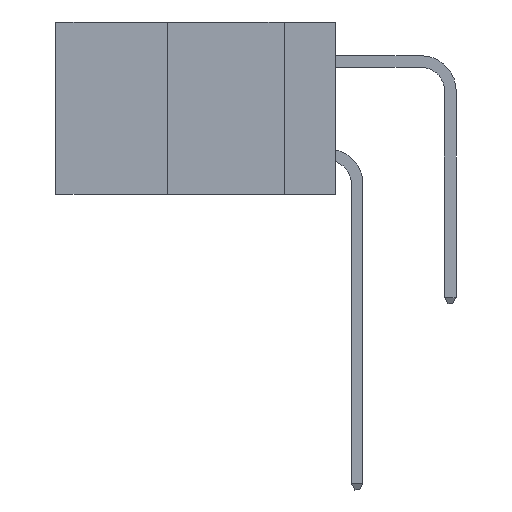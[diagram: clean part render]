
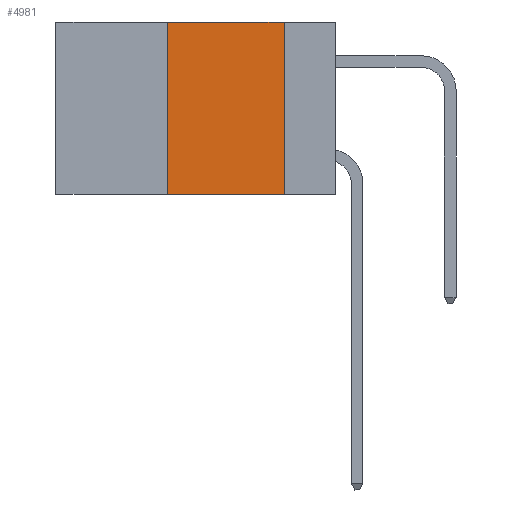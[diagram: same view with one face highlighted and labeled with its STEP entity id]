
A CAD part, left-side view. The second image highlights one B-rep face of the part: STEP entity #4981.
In plain terms, the highlighted planar face has unit normal (-1, 0, 0).
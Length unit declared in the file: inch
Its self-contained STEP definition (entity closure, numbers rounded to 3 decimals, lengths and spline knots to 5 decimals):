
#134 = EDGE_LOOP ( 'NONE', ( #2516, #8405, #8003, #6648 ) ) ;
#233 = DIRECTION ( 'NONE',  ( 0., 0., -1. ) ) ;
#290 = CARTESIAN_POINT ( 'NONE',  ( 0., 0.36, 0. ) ) ;
#1017 = AXIS2_PLACEMENT_3D ( 'NONE', #3306, #8177, #233 ) ;
#1051 = EDGE_CURVE ( 'NONE', #4063, #10425, #11181, .T. ) ;
#1312 = EDGE_CURVE ( 'NONE', #4381, #4063, #7169, .T. ) ;
#1988 = EDGE_CURVE ( 'NONE', #4381, #3620, #2756, .T. ) ;
#2516 = ORIENTED_EDGE ( 'NONE', *, *, #8162, .F. ) ;
#2756 = LINE ( 'NONE', #12346, #5768 ) ;
#2904 = DIRECTION ( 'NONE',  ( 0., -1., 0. ) ) ;
#3306 = CARTESIAN_POINT ( 'NONE',  ( 0., 0.6, 0. ) ) ;
#3620 = VERTEX_POINT ( 'NONE', #7656 ) ;
#4063 = VERTEX_POINT ( 'NONE', #290 ) ;
#4265 = CARTESIAN_POINT ( 'NONE',  ( 0., 0.11, 0. ) ) ;
#4273 = LINE ( 'NONE', #12204, #10775 ) ;
#4381 = VERTEX_POINT ( 'NONE', #11476 ) ;
#4629 = DIRECTION ( 'NONE',  ( 0., 0., -1. ) ) ;
#4711 = CARTESIAN_POINT ( 'NONE',  ( 0., 0.6, 0. ) ) ;
#4981 = ADVANCED_FACE ( 'NONE', ( #7603 ), #5149, .F. ) ;
#5149 = PLANE ( 'NONE',  #1017 ) ;
#5212 = VECTOR ( 'NONE', #10028, 39.37008 ) ;
#5768 = VECTOR ( 'NONE', #10433, 39.37008 ) ;
#6514 = VECTOR ( 'NONE', #2904, 39.37008 ) ;
#6648 = ORIENTED_EDGE ( 'NONE', *, *, #1988, .T. ) ;
#7169 = LINE ( 'NONE', #8035, #5212 ) ;
#7603 = FACE_OUTER_BOUND ( 'NONE', #134, .T. ) ;
#7656 = CARTESIAN_POINT ( 'NONE',  ( 0., 0.11, -0.37 ) ) ;
#8003 = ORIENTED_EDGE ( 'NONE', *, *, #1312, .F. ) ;
#8035 = CARTESIAN_POINT ( 'NONE',  ( 0., 0.36, 0. ) ) ;
#8162 = EDGE_CURVE ( 'NONE', #10425, #3620, #4273, .T. ) ;
#8177 = DIRECTION ( 'NONE',  ( 1., 0., 0. ) ) ;
#8405 = ORIENTED_EDGE ( 'NONE', *, *, #1051, .F. ) ;
#10028 = DIRECTION ( 'NONE',  ( 0., 0., 1. ) ) ;
#10425 = VERTEX_POINT ( 'NONE', #4265 ) ;
#10433 = DIRECTION ( 'NONE',  ( 0., -1., 0. ) ) ;
#10775 = VECTOR ( 'NONE', #4629, 39.37008 ) ;
#11181 = LINE ( 'NONE', #4711, #6514 ) ;
#11476 = CARTESIAN_POINT ( 'NONE',  ( 0., 0.36, -0.37 ) ) ;
#12204 = CARTESIAN_POINT ( 'NONE',  ( 0., 0.11, 0. ) ) ;
#12346 = CARTESIAN_POINT ( 'NONE',  ( 0., 0.6, -0.37 ) ) ;
